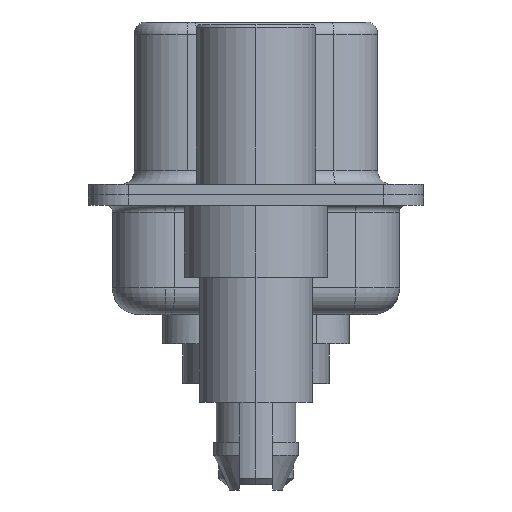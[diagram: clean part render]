
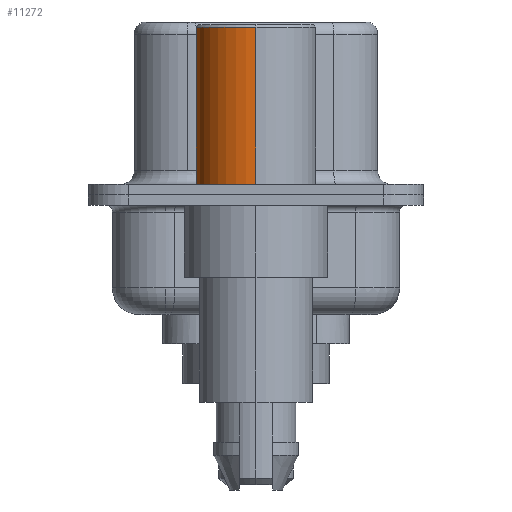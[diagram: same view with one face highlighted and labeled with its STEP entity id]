
A CAD part, left-side view. The second image highlights one B-rep face of the part: STEP entity #11272.
In plain terms, the highlighted cylindrical face has radius 2.25 mm (diameter 4.5 mm), a partial arc.
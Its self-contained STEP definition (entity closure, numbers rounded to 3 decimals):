
#483 = AXIS2_PLACEMENT_3D ( 'NONE', #4886, #4627, #10189 ) ;
#484 = DIRECTION ( 'NONE',  ( 0., 0., 1. ) ) ;
#674 = ORIENTED_EDGE ( 'NONE', *, *, #8784, .F. ) ;
#682 = AXIS2_PLACEMENT_3D ( 'NONE', #7820, #484, #9040 ) ;
#1099 = EDGE_CURVE ( 'NONE', #7381, #7487, #2578, .T. ) ;
#1181 = AXIS2_PLACEMENT_3D ( 'NONE', #6840, #3130, #4355 ) ;
#1526 = ORIENTED_EDGE ( 'NONE', *, *, #3506, .T. ) ;
#1532 = DIRECTION ( 'NONE',  ( 0., 0., 1. ) ) ;
#2399 = CARTESIAN_POINT ( 'NONE',  ( 2.25, 0., 0.4 ) ) ;
#2578 = LINE ( 'NONE', #14184, #15315 ) ;
#2693 = EDGE_LOOP ( 'NONE', ( #1526, #10307, #4424, #674 ) ) ;
#3130 = DIRECTION ( 'NONE',  ( 0., 0., 1. ) ) ;
#3506 = EDGE_CURVE ( 'NONE', #6075, #7381, #15678, .T. ) ;
#3681 = CARTESIAN_POINT ( 'NONE',  ( 2.25, 0., 6.3 ) ) ;
#3821 = CIRCLE ( 'NONE', #682, 2.25 ) ;
#3836 = CARTESIAN_POINT ( 'NONE',  ( 2.25, 0., 0.581 ) ) ;
#4355 = DIRECTION ( 'NONE',  ( 1., 0., 0. ) ) ;
#4424 = ORIENTED_EDGE ( 'NONE', *, *, #13986, .F. ) ;
#4627 = DIRECTION ( 'NONE',  ( 0., 0., 1. ) ) ;
#4886 = CARTESIAN_POINT ( 'NONE',  ( 0., 0., 0.4 ) ) ;
#6075 = VERTEX_POINT ( 'NONE', #2399 ) ;
#6245 = CARTESIAN_POINT ( 'NONE',  ( -2.25, 0., 0.4 ) ) ;
#6508 = CARTESIAN_POINT ( 'NONE',  ( -2.25, 0., 6.3 ) ) ;
#6840 = CARTESIAN_POINT ( 'NONE',  ( 0., 0., 0.581 ) ) ;
#6962 = CYLINDRICAL_SURFACE ( 'NONE', #1181, 2.25 ) ;
#7360 = FACE_OUTER_BOUND ( 'NONE', #2693, .T. ) ;
#7381 = VERTEX_POINT ( 'NONE', #6245 ) ;
#7487 = VERTEX_POINT ( 'NONE', #6508 ) ;
#7820 = CARTESIAN_POINT ( 'NONE',  ( 0., 0., 6.3 ) ) ;
#8744 = VECTOR ( 'NONE', #12401, 1000. ) ;
#8784 = EDGE_CURVE ( 'NONE', #6075, #12784, #15289, .T. ) ;
#9040 = DIRECTION ( 'NONE',  ( 1., 0., 0. ) ) ;
#10189 = DIRECTION ( 'NONE',  ( 1., 0., 0. ) ) ;
#10307 = ORIENTED_EDGE ( 'NONE', *, *, #1099, .T. ) ;
#11272 = ADVANCED_FACE ( 'NONE', ( #7360 ), #6962, .T. ) ;
#12401 = DIRECTION ( 'NONE',  ( 0., 0., 1. ) ) ;
#12784 = VERTEX_POINT ( 'NONE', #3681 ) ;
#13986 = EDGE_CURVE ( 'NONE', #12784, #7487, #3821, .T. ) ;
#14184 = CARTESIAN_POINT ( 'NONE',  ( -2.25, 0., 0.581 ) ) ;
#15289 = LINE ( 'NONE', #3836, #8744 ) ;
#15315 = VECTOR ( 'NONE', #1532, 1000. ) ;
#15678 = CIRCLE ( 'NONE', #483, 2.25 ) ;
